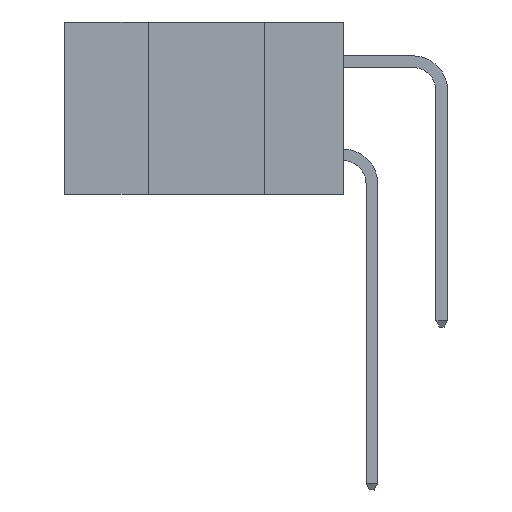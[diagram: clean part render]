
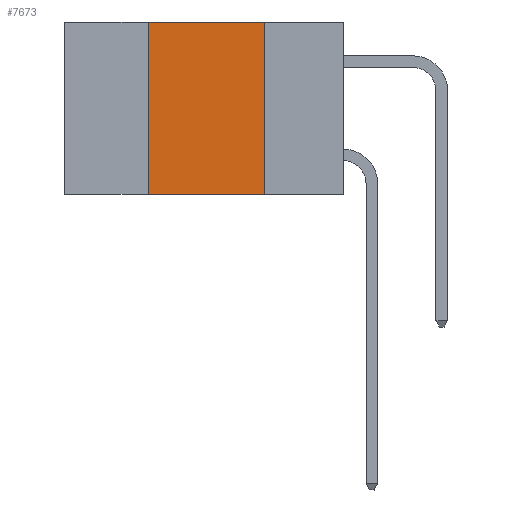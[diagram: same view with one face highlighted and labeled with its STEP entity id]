
A CAD part, left-side view. The second image highlights one B-rep face of the part: STEP entity #7673.
In plain terms, the highlighted planar face has unit normal (-1, 0, 0).
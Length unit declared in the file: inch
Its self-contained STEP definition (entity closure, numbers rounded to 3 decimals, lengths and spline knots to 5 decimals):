
#31 = LINE ( 'NONE', #5123, #166 ) ;
#125 = AXIS2_PLACEMENT_3D ( 'NONE', #4684, #446, #2213 ) ;
#129 = VERTEX_POINT ( 'NONE', #1819 ) ;
#166 = VECTOR ( 'NONE', #6125, 39.37008 ) ;
#219 = CARTESIAN_POINT ( 'NONE',  ( 0., 0.17, 0. ) ) ;
#446 = DIRECTION ( 'NONE',  ( 1., 0., 0. ) ) ;
#1473 = CARTESIAN_POINT ( 'NONE',  ( 0., 0.42, 0. ) ) ;
#1819 = CARTESIAN_POINT ( 'NONE',  ( 0., 0.17, -0.37 ) ) ;
#2070 = EDGE_CURVE ( 'NONE', #10940, #129, #7952, .T. ) ;
#2213 = DIRECTION ( 'NONE',  ( 0., 0., -1. ) ) ;
#2294 = VERTEX_POINT ( 'NONE', #6539 ) ;
#3186 = CARTESIAN_POINT ( 'NONE',  ( 0., 0.42, -0.37 ) ) ;
#3533 = VECTOR ( 'NONE', #10640, 39.37008 ) ;
#3654 = PLANE ( 'NONE',  #125 ) ;
#3793 = ORIENTED_EDGE ( 'NONE', *, *, #8070, .F. ) ;
#3839 = EDGE_LOOP ( 'NONE', ( #6244, #9970, #3793, #4193 ) ) ;
#4098 = FACE_OUTER_BOUND ( 'NONE', #3839, .T. ) ;
#4193 = ORIENTED_EDGE ( 'NONE', *, *, #2070, .T. ) ;
#4684 = CARTESIAN_POINT ( 'NONE',  ( 0., 0.6, 0. ) ) ;
#5123 = CARTESIAN_POINT ( 'NONE',  ( 0., 0.42, 0. ) ) ;
#5124 = EDGE_CURVE ( 'NONE', #2294, #129, #7222, .T. ) ;
#5344 = VECTOR ( 'NONE', #9341, 39.37008 ) ;
#6125 = DIRECTION ( 'NONE',  ( 0., 0., 1. ) ) ;
#6244 = ORIENTED_EDGE ( 'NONE', *, *, #5124, .F. ) ;
#6532 = VERTEX_POINT ( 'NONE', #1473 ) ;
#6539 = CARTESIAN_POINT ( 'NONE',  ( 0., 0.17, 0. ) ) ;
#7023 = EDGE_CURVE ( 'NONE', #6532, #2294, #7819, .T. ) ;
#7222 = LINE ( 'NONE', #219, #3533 ) ;
#7673 = ADVANCED_FACE ( 'NONE', ( #4098 ), #3654, .F. ) ;
#7699 = VECTOR ( 'NONE', #8743, 39.37008 ) ;
#7819 = LINE ( 'NONE', #10996, #5344 ) ;
#7952 = LINE ( 'NONE', #10413, #7699 ) ;
#8070 = EDGE_CURVE ( 'NONE', #10940, #6532, #31, .T. ) ;
#8743 = DIRECTION ( 'NONE',  ( 0., -1., 0. ) ) ;
#9341 = DIRECTION ( 'NONE',  ( 0., -1., 0. ) ) ;
#9970 = ORIENTED_EDGE ( 'NONE', *, *, #7023, .F. ) ;
#10413 = CARTESIAN_POINT ( 'NONE',  ( 0., 0.6, -0.37 ) ) ;
#10640 = DIRECTION ( 'NONE',  ( 0., 0., -1. ) ) ;
#10940 = VERTEX_POINT ( 'NONE', #3186 ) ;
#10996 = CARTESIAN_POINT ( 'NONE',  ( 0., 0.6, 0. ) ) ;
